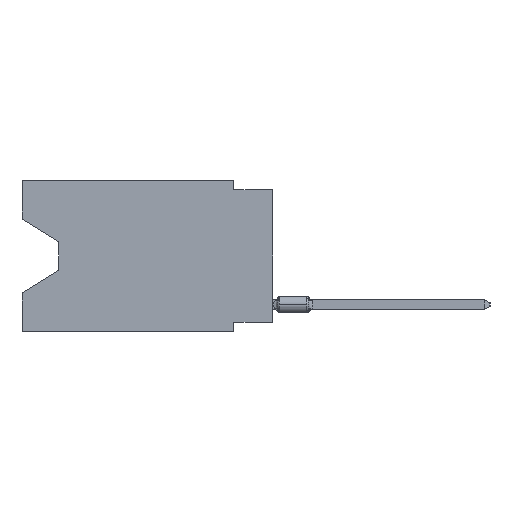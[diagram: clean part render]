
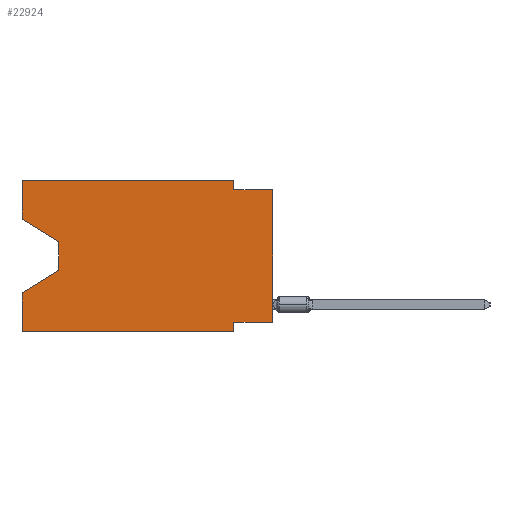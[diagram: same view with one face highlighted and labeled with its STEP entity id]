
A CAD part, left-side view. The second image highlights one B-rep face of the part: STEP entity #22924.
In plain terms, the highlighted planar face has unit normal (-1, 0, 0).
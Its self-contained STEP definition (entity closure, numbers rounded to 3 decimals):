
#480 = ORIENTED_EDGE ( 'NONE', *, *, #35763, .T. ) ;
#492 = CARTESIAN_POINT ( 'NONE',  ( 0., 16.383, -2.546 ) ) ;
#561 = FACE_OUTER_BOUND ( 'NONE', #34092, .T. ) ;
#1866 = VERTEX_POINT ( 'NONE', #58936 ) ;
#3668 = EDGE_CURVE ( 'NONE', #4144, #19796, #13052, .T. ) ;
#3778 = LINE ( 'NONE', #32275, #8673 ) ;
#4144 = VERTEX_POINT ( 'NONE', #21114 ) ;
#4358 = CARTESIAN_POINT ( 'NONE',  ( 0., 2.54, 0. ) ) ;
#4661 = DIRECTION ( 'NONE',  ( 0., -1., 0. ) ) ;
#5973 = PLANE ( 'NONE',  #19899 ) ;
#7792 = VECTOR ( 'NONE', #17182, 1000. ) ;
#8248 = DIRECTION ( 'NONE',  ( 0., 0., -1. ) ) ;
#8673 = VECTOR ( 'NONE', #4661, 1000. ) ;
#10607 = CARTESIAN_POINT ( 'NONE',  ( 0., 13.97, -4.013 ) ) ;
#11651 = DIRECTION ( 'NONE',  ( 0., 0., 1. ) ) ;
#13052 = LINE ( 'NONE', #48814, #17875 ) ;
#13445 = VECTOR ( 'NONE', #26579, 1000. ) ;
#14269 = VERTEX_POINT ( 'NONE', #34374 ) ;
#14849 = CARTESIAN_POINT ( 'NONE',  ( 0., 2.54, -0.635 ) ) ;
#15347 = VECTOR ( 'NONE', #11651, 1000. ) ;
#15705 = DIRECTION ( 'NONE',  ( 0., 0., -1. ) ) ;
#16924 = CARTESIAN_POINT ( 'NONE',  ( 0., 16.383, 0. ) ) ;
#17056 = VECTOR ( 'NONE', #27851, 1000. ) ;
#17182 = DIRECTION ( 'NONE',  ( 0., 1., 0. ) ) ;
#17220 = CARTESIAN_POINT ( 'NONE',  ( 0., 0., -0.635 ) ) ;
#17316 = ORIENTED_EDGE ( 'NONE', *, *, #53655, .T. ) ;
#17875 = VECTOR ( 'NONE', #8248, 1000. ) ;
#18083 = LINE ( 'NONE', #36394, #7792 ) ;
#19303 = CARTESIAN_POINT ( 'NONE',  ( 0., 2.54, 0. ) ) ;
#19409 = VECTOR ( 'NONE', #15705, 1000. ) ;
#19796 = VERTEX_POINT ( 'NONE', #43032 ) ;
#19899 = AXIS2_PLACEMENT_3D ( 'NONE', #24552, #55202, #51610 ) ;
#20838 = DIRECTION ( 'NONE',  ( 0., 0., 1. ) ) ;
#21114 = CARTESIAN_POINT ( 'NONE',  ( 0., 2.54, -9.271 ) ) ;
#21138 = LINE ( 'NONE', #48481, #58486 ) ;
#22924 = ADVANCED_FACE ( 'NONE', ( #561 ), #5973, .F. ) ;
#23431 = VERTEX_POINT ( 'NONE', #10607 ) ;
#24552 = CARTESIAN_POINT ( 'NONE',  ( 0., 16.383, 0. ) ) ;
#24768 = VECTOR ( 'NONE', #40491, 1000. ) ;
#25430 = EDGE_CURVE ( 'NONE', #54152, #55528, #33574, .T. ) ;
#25763 = CARTESIAN_POINT ( 'NONE',  ( 0., 16.383, 0. ) ) ;
#25978 = EDGE_CURVE ( 'NONE', #57952, #1866, #43969, .T. ) ;
#26579 = DIRECTION ( 'NONE',  ( 0., 0., -1. ) ) ;
#26816 = DIRECTION ( 'NONE',  ( 0., -0.855, -0.519 ) ) ;
#26967 = LINE ( 'NONE', #45583, #17056 ) ;
#27350 = ORIENTED_EDGE ( 'NONE', *, *, #47054, .T. ) ;
#27851 = DIRECTION ( 'NONE',  ( 0., 0.855, -0.519 ) ) ;
#28642 = VERTEX_POINT ( 'NONE', #16924 ) ;
#28782 = ORIENTED_EDGE ( 'NONE', *, *, #43857, .F. ) ;
#29502 = LINE ( 'NONE', #38535, #19409 ) ;
#32198 = VERTEX_POINT ( 'NONE', #492 ) ;
#32275 = CARTESIAN_POINT ( 'NONE',  ( 0., 16.383, -9.906 ) ) ;
#33574 = LINE ( 'NONE', #47116, #15347 ) ;
#34092 = EDGE_LOOP ( 'NONE', ( #17316, #27350, #42955, #37973, #480, #39000, #28782, #51940, #36078, #52251, #39513, #42126 ) ) ;
#34374 = CARTESIAN_POINT ( 'NONE',  ( 0., 13.97, -5.893 ) ) ;
#35763 = EDGE_CURVE ( 'NONE', #54152, #19796, #3778, .T. ) ;
#36078 = ORIENTED_EDGE ( 'NONE', *, *, #25978, .F. ) ;
#36394 = CARTESIAN_POINT ( 'NONE',  ( 0., 0., -9.271 ) ) ;
#37522 = VERTEX_POINT ( 'NONE', #49443 ) ;
#37973 = ORIENTED_EDGE ( 'NONE', *, *, #25430, .F. ) ;
#38058 = EDGE_CURVE ( 'NONE', #14269, #55528, #26967, .T. ) ;
#38535 = CARTESIAN_POINT ( 'NONE',  ( 0., 13.97, -4.013 ) ) ;
#39000 = ORIENTED_EDGE ( 'NONE', *, *, #3668, .F. ) ;
#39513 = ORIENTED_EDGE ( 'NONE', *, *, #51668, .F. ) ;
#40366 = DIRECTION ( 'NONE',  ( 0., -1., 0. ) ) ;
#40491 = DIRECTION ( 'NONE',  ( 0., -1., 0. ) ) ;
#41204 = CARTESIAN_POINT ( 'NONE',  ( 0., 16.383, 0. ) ) ;
#42126 = ORIENTED_EDGE ( 'NONE', *, *, #43882, .F. ) ;
#42229 = VECTOR ( 'NONE', #26816, 1000. ) ;
#42416 = DIRECTION ( 'NONE',  ( 0., 0., 1. ) ) ;
#42698 = EDGE_CURVE ( 'NONE', #56760, #57952, #49717, .T. ) ;
#42871 = EDGE_CURVE ( 'NONE', #37522, #1866, #21138, .T. ) ;
#42955 = ORIENTED_EDGE ( 'NONE', *, *, #38058, .T. ) ;
#43032 = CARTESIAN_POINT ( 'NONE',  ( 0., 2.54, -9.906 ) ) ;
#43857 = EDGE_CURVE ( 'NONE', #37522, #4144, #18083, .T. ) ;
#43882 = EDGE_CURVE ( 'NONE', #32198, #28642, #47233, .T. ) ;
#43969 = LINE ( 'NONE', #17220, #49902 ) ;
#45583 = CARTESIAN_POINT ( 'NONE',  ( 0., 13.97, -5.893 ) ) ;
#47054 = EDGE_CURVE ( 'NONE', #23431, #14269, #29502, .T. ) ;
#47116 = CARTESIAN_POINT ( 'NONE',  ( 0., 16.383, 0. ) ) ;
#47233 = LINE ( 'NONE', #41204, #48063 ) ;
#48063 = VECTOR ( 'NONE', #42416, 1000. ) ;
#48481 = CARTESIAN_POINT ( 'NONE',  ( 0., 0., 0. ) ) ;
#48488 = CARTESIAN_POINT ( 'NONE',  ( 0., 16.383, -2.546 ) ) ;
#48777 = LINE ( 'NONE', #48488, #42229 ) ;
#48814 = CARTESIAN_POINT ( 'NONE',  ( 0., 2.54, -9.906 ) ) ;
#49443 = CARTESIAN_POINT ( 'NONE',  ( 0., 0., -9.271 ) ) ;
#49717 = LINE ( 'NONE', #4358, #13445 ) ;
#49902 = VECTOR ( 'NONE', #40366, 1000. ) ;
#50819 = CARTESIAN_POINT ( 'NONE',  ( 0., 16.383, -7.36 ) ) ;
#51610 = DIRECTION ( 'NONE',  ( 0., 0., -1. ) ) ;
#51668 = EDGE_CURVE ( 'NONE', #28642, #56760, #54305, .T. ) ;
#51940 = ORIENTED_EDGE ( 'NONE', *, *, #42871, .T. ) ;
#52251 = ORIENTED_EDGE ( 'NONE', *, *, #42698, .F. ) ;
#52656 = CARTESIAN_POINT ( 'NONE',  ( 0., 16.383, -9.906 ) ) ;
#53655 = EDGE_CURVE ( 'NONE', #32198, #23431, #48777, .T. ) ;
#54152 = VERTEX_POINT ( 'NONE', #52656 ) ;
#54305 = LINE ( 'NONE', #25763, #24768 ) ;
#55202 = DIRECTION ( 'NONE',  ( 1., 0., 0. ) ) ;
#55528 = VERTEX_POINT ( 'NONE', #50819 ) ;
#56760 = VERTEX_POINT ( 'NONE', #19303 ) ;
#57952 = VERTEX_POINT ( 'NONE', #14849 ) ;
#58486 = VECTOR ( 'NONE', #20838, 1000. ) ;
#58936 = CARTESIAN_POINT ( 'NONE',  ( 0., 0., -0.635 ) ) ;
